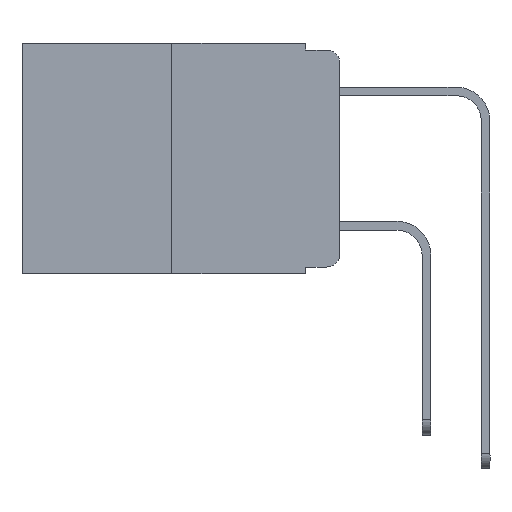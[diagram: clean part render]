
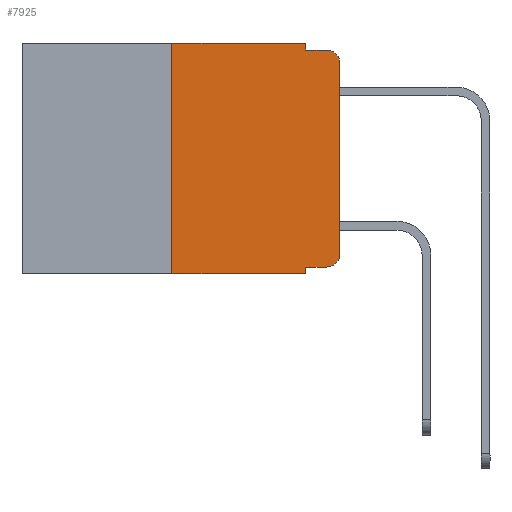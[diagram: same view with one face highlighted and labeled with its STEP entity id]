
A CAD part, left-side view. The second image highlights one B-rep face of the part: STEP entity #7925.
In plain terms, the highlighted planar face has unit normal (-1, 0, 0).
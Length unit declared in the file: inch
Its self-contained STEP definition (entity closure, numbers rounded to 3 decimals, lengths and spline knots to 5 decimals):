
#264 = LINE ( 'NONE', #4894, #2399 ) ;
#633 = EDGE_CURVE ( 'NONE', #10101, #6141, #14253, .T. ) ;
#828 = LINE ( 'NONE', #6691, #12252 ) ;
#967 = ORIENTED_EDGE ( 'NONE', *, *, #13281, .T. ) ;
#1128 = DIRECTION ( 'NONE',  ( 1., 0., 0. ) ) ;
#1770 = CARTESIAN_POINT ( 'NONE',  ( 0., 0.02, -0.03 ) ) ;
#2399 = VECTOR ( 'NONE', #8491, 39.37008 ) ;
#2409 = VERTEX_POINT ( 'NONE', #8687 ) ;
#2477 = LINE ( 'NONE', #5661, #5361 ) ;
#2531 = EDGE_CURVE ( 'NONE', #7666, #6333, #828, .T. ) ;
#2794 = CARTESIAN_POINT ( 'NONE',  ( 0., 0.051, -0.01 ) ) ;
#3095 = LINE ( 'NONE', #11322, #7548 ) ;
#3541 = FACE_OUTER_BOUND ( 'NONE', #3604, .T. ) ;
#3604 = EDGE_LOOP ( 'NONE', ( #10699, #7453, #13200, #4601, #9918, #4543, #5945, #5653, #13753, #967 ) ) ;
#3666 = VERTEX_POINT ( 'NONE', #5508 ) ;
#4098 = VERTEX_POINT ( 'NONE', #9937 ) ;
#4157 = VECTOR ( 'NONE', #5246, 39.37008 ) ;
#4179 = DIRECTION ( 'NONE',  ( 0., 0., -1. ) ) ;
#4529 = EDGE_CURVE ( 'NONE', #3666, #6333, #10563, .T. ) ;
#4543 = ORIENTED_EDGE ( 'NONE', *, *, #6294, .F. ) ;
#4601 = ORIENTED_EDGE ( 'NONE', *, *, #12214, .F. ) ;
#4894 = CARTESIAN_POINT ( 'NONE',  ( 0., 0., 0. ) ) ;
#5066 = VECTOR ( 'NONE', #7550, 39.37008 ) ;
#5114 = DIRECTION ( 'NONE',  ( -1., 0., 0. ) ) ;
#5246 = DIRECTION ( 'NONE',  ( 0., -1., 0. ) ) ;
#5361 = VECTOR ( 'NONE', #7049, 39.37008 ) ;
#5508 = CARTESIAN_POINT ( 'NONE',  ( 0., 0., -0.03 ) ) ;
#5653 = ORIENTED_EDGE ( 'NONE', *, *, #8178, .F. ) ;
#5661 = CARTESIAN_POINT ( 'NONE',  ( 0., 0.051, -0.333 ) ) ;
#5945 = ORIENTED_EDGE ( 'NONE', *, *, #13405, .T. ) ;
#6128 = CIRCLE ( 'NONE', #8315, 0.02 ) ;
#6141 = VERTEX_POINT ( 'NONE', #12313 ) ;
#6294 = EDGE_CURVE ( 'NONE', #10817, #10101, #8980, .T. ) ;
#6333 = VERTEX_POINT ( 'NONE', #11477 ) ;
#6691 = CARTESIAN_POINT ( 'NONE',  ( 0., 0.051, -0.01 ) ) ;
#7049 = DIRECTION ( 'NONE',  ( 0., -1., 0. ) ) ;
#7453 = ORIENTED_EDGE ( 'NONE', *, *, #4529, .T. ) ;
#7477 = LINE ( 'NONE', #12109, #4157 ) ;
#7548 = VECTOR ( 'NONE', #9050, 39.37008 ) ;
#7550 = DIRECTION ( 'NONE',  ( 0., -1., 0. ) ) ;
#7573 = CARTESIAN_POINT ( 'NONE',  ( 0., 0., -0.313 ) ) ;
#7666 = VERTEX_POINT ( 'NONE', #2794 ) ;
#7823 = DIRECTION ( 'NONE',  ( 0., -1., 0. ) ) ;
#7849 = CARTESIAN_POINT ( 'NONE',  ( 0., 0.25, 0. ) ) ;
#7907 = CARTESIAN_POINT ( 'NONE',  ( 0., 0.25, 0. ) ) ;
#7925 = ADVANCED_FACE ( 'NONE', ( #3541 ), #11692, .F. ) ;
#8178 = EDGE_CURVE ( 'NONE', #4098, #12877, #12984, .T. ) ;
#8228 = VECTOR ( 'NONE', #14208, 39.37008 ) ;
#8315 = AXIS2_PLACEMENT_3D ( 'NONE', #14553, #13336, #8633 ) ;
#8491 = DIRECTION ( 'NONE',  ( 0., 0., 1. ) ) ;
#8586 = EDGE_CURVE ( 'NONE', #14228, #3666, #264, .T. ) ;
#8633 = DIRECTION ( 'NONE',  ( 0., 0., -1. ) ) ;
#8687 = CARTESIAN_POINT ( 'NONE',  ( 0., 0.02, -0.333 ) ) ;
#8980 = LINE ( 'NONE', #7907, #12796 ) ;
#9050 = DIRECTION ( 'NONE',  ( 0., 0., -1. ) ) ;
#9494 = CARTESIAN_POINT ( 'NONE',  ( 0., 0.051, -0.343 ) ) ;
#9573 = CARTESIAN_POINT ( 'NONE',  ( 0., 0.051, 0. ) ) ;
#9918 = ORIENTED_EDGE ( 'NONE', *, *, #633, .F. ) ;
#9937 = CARTESIAN_POINT ( 'NONE',  ( 0., 0.051, -0.333 ) ) ;
#10101 = VERTEX_POINT ( 'NONE', #7849 ) ;
#10273 = DIRECTION ( 'NONE',  ( 0., 0., 1. ) ) ;
#10333 = DIRECTION ( 'NONE',  ( 0., 0., -1. ) ) ;
#10402 = AXIS2_PLACEMENT_3D ( 'NONE', #11536, #1128, #10333 ) ;
#10563 = CIRCLE ( 'NONE', #13476, 0.02 ) ;
#10699 = ORIENTED_EDGE ( 'NONE', *, *, #8586, .T. ) ;
#10817 = VERTEX_POINT ( 'NONE', #11936 ) ;
#11322 = CARTESIAN_POINT ( 'NONE',  ( 0., 0.051, 0. ) ) ;
#11477 = CARTESIAN_POINT ( 'NONE',  ( 0., 0.02, -0.01 ) ) ;
#11536 = CARTESIAN_POINT ( 'NONE',  ( 0., 0.473, 0. ) ) ;
#11692 = PLANE ( 'NONE',  #10402 ) ;
#11936 = CARTESIAN_POINT ( 'NONE',  ( 0., 0.25, -0.343 ) ) ;
#12109 = CARTESIAN_POINT ( 'NONE',  ( 0., 0.473, -0.343 ) ) ;
#12214 = EDGE_CURVE ( 'NONE', #6141, #7666, #3095, .T. ) ;
#12252 = VECTOR ( 'NONE', #7823, 39.37008 ) ;
#12313 = CARTESIAN_POINT ( 'NONE',  ( 0., 0.051, 0. ) ) ;
#12685 = EDGE_CURVE ( 'NONE', #4098, #2409, #2477, .T. ) ;
#12796 = VECTOR ( 'NONE', #10273, 39.37008 ) ;
#12877 = VERTEX_POINT ( 'NONE', #9494 ) ;
#12984 = LINE ( 'NONE', #9573, #8228 ) ;
#13200 = ORIENTED_EDGE ( 'NONE', *, *, #2531, .F. ) ;
#13281 = EDGE_CURVE ( 'NONE', #2409, #14228, #6128, .T. ) ;
#13335 = CARTESIAN_POINT ( 'NONE',  ( 0., 0.473, 0. ) ) ;
#13336 = DIRECTION ( 'NONE',  ( -1., 0., 0. ) ) ;
#13405 = EDGE_CURVE ( 'NONE', #10817, #12877, #7477, .T. ) ;
#13476 = AXIS2_PLACEMENT_3D ( 'NONE', #1770, #5114, #4179 ) ;
#13753 = ORIENTED_EDGE ( 'NONE', *, *, #12685, .T. ) ;
#14208 = DIRECTION ( 'NONE',  ( 0., 0., -1. ) ) ;
#14228 = VERTEX_POINT ( 'NONE', #7573 ) ;
#14253 = LINE ( 'NONE', #13335, #5066 ) ;
#14553 = CARTESIAN_POINT ( 'NONE',  ( 0., 0.02, -0.313 ) ) ;
